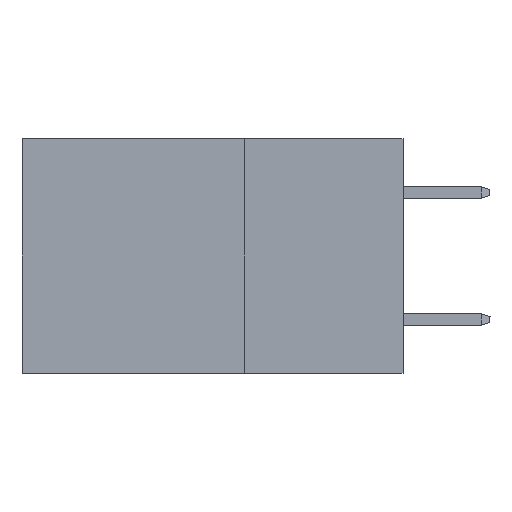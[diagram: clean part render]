
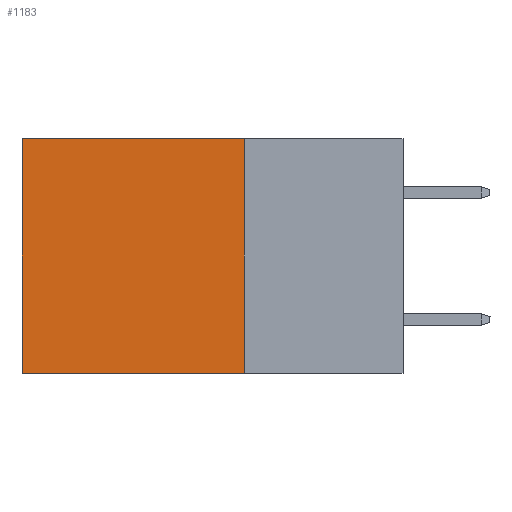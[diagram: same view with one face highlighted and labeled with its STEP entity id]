
A CAD part, left-side view. The second image highlights one B-rep face of the part: STEP entity #1183.
In plain terms, the highlighted planar face has unit normal (-1, 0, 0).
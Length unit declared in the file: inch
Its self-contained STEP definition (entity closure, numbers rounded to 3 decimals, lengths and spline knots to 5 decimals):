
#1183 = ADVANCED_FACE ( 'NONE', ( #11665 ), #4520, .F. ) ;
#2392 = DIRECTION ( 'NONE',  ( 1., 0., 0. ) ) ;
#3423 = LINE ( 'NONE', #26533, #24511 ) ;
#3782 = LINE ( 'NONE', #25231, #6943 ) ;
#4520 = PLANE ( 'NONE',  #23900 ) ;
#4573 = EDGE_CURVE ( 'NONE', #15777, #21911, #3423, .T. ) ;
#6420 = ORIENTED_EDGE ( 'NONE', *, *, #4573, .T. ) ;
#6943 = VECTOR ( 'NONE', #22095, 39.37008 ) ;
#11665 = FACE_OUTER_BOUND ( 'NONE', #17682, .T. ) ;
#14607 = VECTOR ( 'NONE', #29880, 39.37008 ) ;
#15517 = CARTESIAN_POINT ( 'NONE',  ( 0.2875, 0.6, -0.37 ) ) ;
#15777 = VERTEX_POINT ( 'NONE', #34572 ) ;
#17218 = CARTESIAN_POINT ( 'NONE',  ( 0.2875, 0.25, 0. ) ) ;
#17271 = CARTESIAN_POINT ( 'NONE',  ( 0.2875, 0.25, 0. ) ) ;
#17682 = EDGE_LOOP ( 'NONE', ( #6420, #36581, #21279, #29158 ) ) ;
#21279 = ORIENTED_EDGE ( 'NONE', *, *, #36632, .F. ) ;
#21561 = EDGE_CURVE ( 'NONE', #26822, #15777, #33184, .T. ) ;
#21911 = VERTEX_POINT ( 'NONE', #15517 ) ;
#22095 = DIRECTION ( 'NONE',  ( 0., 1., 0. ) ) ;
#23312 = VECTOR ( 'NONE', #36537, 39.37008 ) ;
#23900 = AXIS2_PLACEMENT_3D ( 'NONE', #25507, #2392, #40866 ) ;
#24511 = VECTOR ( 'NONE', #32442, 39.37008 ) ;
#25231 = CARTESIAN_POINT ( 'NONE',  ( 0.2875, 0.25, -0.37 ) ) ;
#25507 = CARTESIAN_POINT ( 'NONE',  ( 0.2875, 0.25, 0. ) ) ;
#26227 = CARTESIAN_POINT ( 'NONE',  ( 0.2875, 0.25, -0.37 ) ) ;
#26308 = VERTEX_POINT ( 'NONE', #26227 ) ;
#26533 = CARTESIAN_POINT ( 'NONE',  ( 0.2875, 0.6, 0. ) ) ;
#26822 = VERTEX_POINT ( 'NONE', #30374 ) ;
#29158 = ORIENTED_EDGE ( 'NONE', *, *, #21561, .T. ) ;
#29880 = DIRECTION ( 'NONE',  ( 0., 0., -1. ) ) ;
#30374 = CARTESIAN_POINT ( 'NONE',  ( 0.2875, 0.25, 0. ) ) ;
#30426 = EDGE_CURVE ( 'NONE', #26308, #21911, #3782, .T. ) ;
#32442 = DIRECTION ( 'NONE',  ( 0., 0., -1. ) ) ;
#33184 = LINE ( 'NONE', #17218, #23312 ) ;
#33237 = LINE ( 'NONE', #17271, #14607 ) ;
#34572 = CARTESIAN_POINT ( 'NONE',  ( 0.2875, 0.6, 0. ) ) ;
#36537 = DIRECTION ( 'NONE',  ( 0., 1., 0. ) ) ;
#36581 = ORIENTED_EDGE ( 'NONE', *, *, #30426, .F. ) ;
#36632 = EDGE_CURVE ( 'NONE', #26822, #26308, #33237, .T. ) ;
#40866 = DIRECTION ( 'NONE',  ( 0., 0., -1. ) ) ;
